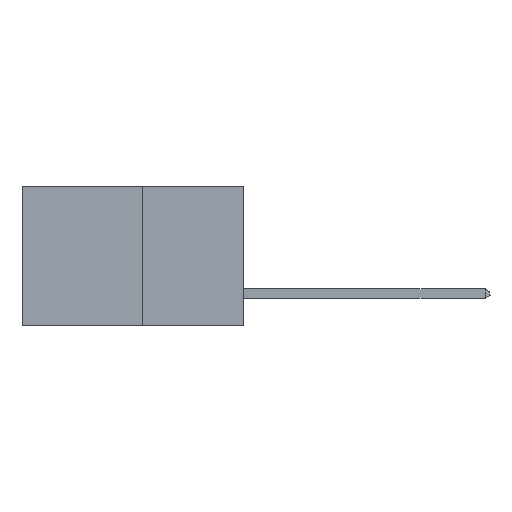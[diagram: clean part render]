
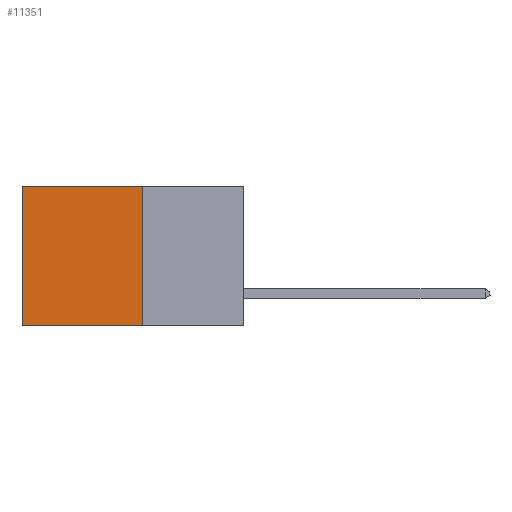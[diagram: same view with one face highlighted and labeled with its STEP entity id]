
A CAD part, left-side view. The second image highlights one B-rep face of the part: STEP entity #11351.
In plain terms, the highlighted planar face has unit normal (-1, 0, 0).
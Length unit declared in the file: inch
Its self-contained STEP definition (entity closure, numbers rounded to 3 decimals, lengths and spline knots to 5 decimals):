
#316 = EDGE_CURVE ( 'NONE', #11056, #5387, #8162, .T. ) ;
#511 = FACE_OUTER_BOUND ( 'NONE', #6359, .T. ) ;
#757 = LINE ( 'NONE', #4224, #9749 ) ;
#948 = VECTOR ( 'NONE', #11344, 39.37008 ) ;
#1145 = DIRECTION ( 'NONE',  ( 0., 0., -1. ) ) ;
#1791 = VERTEX_POINT ( 'NONE', #3096 ) ;
#2643 = ORIENTED_EDGE ( 'NONE', *, *, #10392, .F. ) ;
#2837 = PLANE ( 'NONE',  #6854 ) ;
#3000 = EDGE_CURVE ( 'NONE', #1791, #11056, #7776, .T. ) ;
#3020 = VECTOR ( 'NONE', #7140, 39.37008 ) ;
#3096 = CARTESIAN_POINT ( 'NONE',  ( 0.277, 0.27, 0. ) ) ;
#3710 = DIRECTION ( 'NONE',  ( 1., 0., 0. ) ) ;
#4224 = CARTESIAN_POINT ( 'NONE',  ( 0.277, 0.27, -0.37 ) ) ;
#4855 = CARTESIAN_POINT ( 'NONE',  ( 0.277, 0.59, -0.37 ) ) ;
#5033 = CARTESIAN_POINT ( 'NONE',  ( 0.277, 0.59, 0. ) ) ;
#5059 = VERTEX_POINT ( 'NONE', #8728 ) ;
#5387 = VERTEX_POINT ( 'NONE', #10016 ) ;
#6359 = EDGE_LOOP ( 'NONE', ( #10422, #2643, #6944, #11521 ) ) ;
#6854 = AXIS2_PLACEMENT_3D ( 'NONE', #9103, #3710, #9936 ) ;
#6944 = ORIENTED_EDGE ( 'NONE', *, *, #7784, .F. ) ;
#7140 = DIRECTION ( 'NONE',  ( 0., 1., 0. ) ) ;
#7166 = CARTESIAN_POINT ( 'NONE',  ( 0.277, 0.27, 0. ) ) ;
#7776 = LINE ( 'NONE', #7166, #3020 ) ;
#7784 = EDGE_CURVE ( 'NONE', #1791, #5059, #10256, .T. ) ;
#8162 = LINE ( 'NONE', #4855, #948 ) ;
#8728 = CARTESIAN_POINT ( 'NONE',  ( 0.277, 0.27, -0.37 ) ) ;
#9103 = CARTESIAN_POINT ( 'NONE',  ( 0.277, 0.27, -0.37 ) ) ;
#9588 = DIRECTION ( 'NONE',  ( 0., 1., 0. ) ) ;
#9749 = VECTOR ( 'NONE', #9588, 39.37008 ) ;
#9936 = DIRECTION ( 'NONE',  ( 0., 0., -1. ) ) ;
#9971 = VECTOR ( 'NONE', #1145, 39.37008 ) ;
#10016 = CARTESIAN_POINT ( 'NONE',  ( 0.277, 0.59, -0.37 ) ) ;
#10256 = LINE ( 'NONE', #10939, #9971 ) ;
#10392 = EDGE_CURVE ( 'NONE', #5059, #5387, #757, .T. ) ;
#10422 = ORIENTED_EDGE ( 'NONE', *, *, #316, .T. ) ;
#10939 = CARTESIAN_POINT ( 'NONE',  ( 0.277, 0.27, -0.37 ) ) ;
#11056 = VERTEX_POINT ( 'NONE', #5033 ) ;
#11344 = DIRECTION ( 'NONE',  ( 0., 0., -1. ) ) ;
#11351 = ADVANCED_FACE ( 'NONE', ( #511 ), #2837, .F. ) ;
#11521 = ORIENTED_EDGE ( 'NONE', *, *, #3000, .T. ) ;
